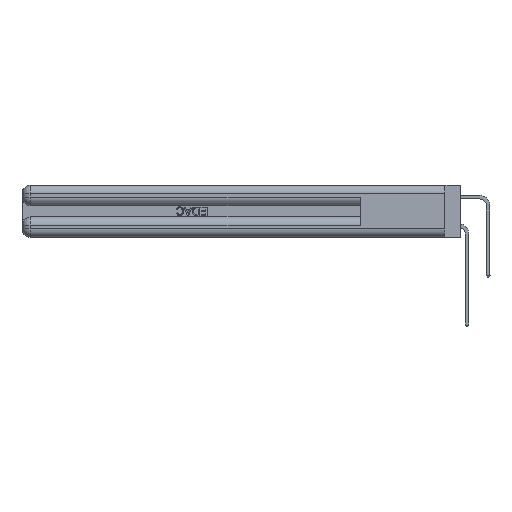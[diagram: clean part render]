
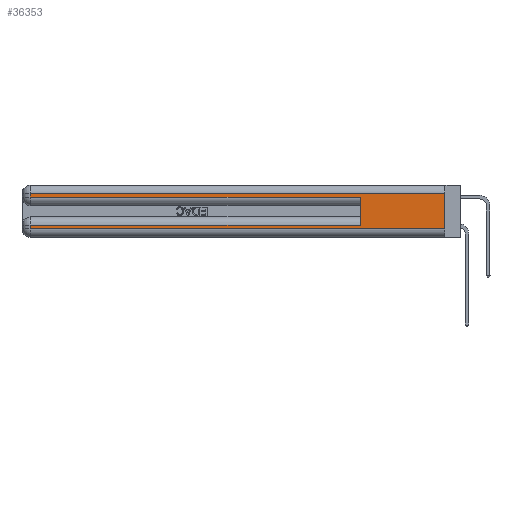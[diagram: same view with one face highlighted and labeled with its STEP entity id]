
A CAD part, left-side view. The second image highlights one B-rep face of the part: STEP entity #36353.
In plain terms, the highlighted planar face has unit normal (-1, 0, 0).
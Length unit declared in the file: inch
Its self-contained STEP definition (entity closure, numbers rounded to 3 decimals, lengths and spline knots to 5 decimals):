
#193 = CARTESIAN_POINT ( 'NONE',  ( 0., 0., 0.285 ) ) ;
#205 = EDGE_CURVE ( 'NONE', #13662, #18976, #2060, .T. ) ;
#457 = EDGE_CURVE ( 'NONE', #8145, #7969, #22100, .T. ) ;
#627 = DIRECTION ( 'NONE',  ( 0., 0., -1. ) ) ;
#692 = CARTESIAN_POINT ( 'NONE',  ( 0., 2.94, 0.37 ) ) ;
#2060 = LINE ( 'NONE', #39021, #38018 ) ;
#2291 = EDGE_CURVE ( 'NONE', #34204, #13143, #17756, .T. ) ;
#3431 = LINE ( 'NONE', #31493, #22983 ) ;
#3568 = LINE ( 'NONE', #34384, #14178 ) ;
#5233 = ORIENTED_EDGE ( 'NONE', *, *, #41923, .T. ) ;
#5401 = ORIENTED_EDGE ( 'NONE', *, *, #205, .T. ) ;
#5977 = DIRECTION ( 'NONE',  ( 0., 0., -1. ) ) ;
#6338 = ORIENTED_EDGE ( 'NONE', *, *, #2291, .F. ) ;
#6559 = EDGE_LOOP ( 'NONE', ( #21436, #18140, #39024, #5233, #6338, #36258, #5401, #8361 ) ) ;
#7005 = DIRECTION ( 'NONE',  ( 0., 1., 0. ) ) ;
#7896 = LINE ( 'NONE', #692, #8948 ) ;
#7969 = VERTEX_POINT ( 'NONE', #29337 ) ;
#8145 = VERTEX_POINT ( 'NONE', #39425 ) ;
#8361 = ORIENTED_EDGE ( 'NONE', *, *, #10549, .T. ) ;
#8948 = VECTOR ( 'NONE', #37995, 39.37008 ) ;
#9521 = CARTESIAN_POINT ( 'NONE',  ( 0., 0., 0.37 ) ) ;
#9901 = CARTESIAN_POINT ( 'NONE',  ( 0., 0.6, 0.145 ) ) ;
#10384 = FACE_OUTER_BOUND ( 'NONE', #6559, .T. ) ;
#10549 = EDGE_CURVE ( 'NONE', #18976, #26614, #3431, .T. ) ;
#13143 = VERTEX_POINT ( 'NONE', #22701 ) ;
#13662 = VERTEX_POINT ( 'NONE', #36046 ) ;
#14178 = VECTOR ( 'NONE', #7005, 39.37008 ) ;
#15717 = AXIS2_PLACEMENT_3D ( 'NONE', #9521, #23370, #5977 ) ;
#16528 = EDGE_CURVE ( 'NONE', #8145, #26614, #27671, .T. ) ;
#17756 = LINE ( 'NONE', #9901, #34706 ) ;
#18140 = ORIENTED_EDGE ( 'NONE', *, *, #457, .T. ) ;
#18976 = VERTEX_POINT ( 'NONE', #35636 ) ;
#19395 = EDGE_CURVE ( 'NONE', #7969, #34662, #7896, .T. ) ;
#19856 = EDGE_CURVE ( 'NONE', #34204, #13662, #3568, .T. ) ;
#21436 = ORIENTED_EDGE ( 'NONE', *, *, #16528, .F. ) ;
#21649 = CARTESIAN_POINT ( 'NONE',  ( 0., 0., 0.06 ) ) ;
#22033 = VECTOR ( 'NONE', #23367, 39.37008 ) ;
#22100 = LINE ( 'NONE', #36299, #41698 ) ;
#22149 = CARTESIAN_POINT ( 'NONE',  ( 0., 0., 0.37 ) ) ;
#22701 = CARTESIAN_POINT ( 'NONE',  ( 0., 0.6, 0.285 ) ) ;
#22983 = VECTOR ( 'NONE', #38126, 39.37008 ) ;
#23367 = DIRECTION ( 'NONE',  ( 0., -1., 0. ) ) ;
#23370 = DIRECTION ( 'NONE',  ( 1., 0., 0. ) ) ;
#26427 = DIRECTION ( 'NONE',  ( 0., 1., 0. ) ) ;
#26614 = VERTEX_POINT ( 'NONE', #21649 ) ;
#27671 = LINE ( 'NONE', #22149, #40911 ) ;
#28400 = LINE ( 'NONE', #193, #22033 ) ;
#29337 = CARTESIAN_POINT ( 'NONE',  ( 0., 2.94, 0.31 ) ) ;
#31493 = CARTESIAN_POINT ( 'NONE',  ( 0., 0., 0.06 ) ) ;
#31574 = CARTESIAN_POINT ( 'NONE',  ( 0., 0.6, 0.085 ) ) ;
#33456 = DIRECTION ( 'NONE',  ( 0., 0., 1. ) ) ;
#34204 = VERTEX_POINT ( 'NONE', #31574 ) ;
#34320 = CARTESIAN_POINT ( 'NONE',  ( 0., 2.94, 0.285 ) ) ;
#34384 = CARTESIAN_POINT ( 'NONE',  ( 0., 0., 0.085 ) ) ;
#34662 = VERTEX_POINT ( 'NONE', #34320 ) ;
#34706 = VECTOR ( 'NONE', #33456, 39.37008 ) ;
#35636 = CARTESIAN_POINT ( 'NONE',  ( 0., 2.94, 0.06 ) ) ;
#36046 = CARTESIAN_POINT ( 'NONE',  ( 0., 2.94, 0.085 ) ) ;
#36258 = ORIENTED_EDGE ( 'NONE', *, *, #19856, .T. ) ;
#36299 = CARTESIAN_POINT ( 'NONE',  ( 0., 0., 0.31 ) ) ;
#36353 = ADVANCED_FACE ( 'NONE', ( #10384 ), #36671, .F. ) ;
#36671 = PLANE ( 'NONE',  #15717 ) ;
#37995 = DIRECTION ( 'NONE',  ( 0., 0., -1. ) ) ;
#38018 = VECTOR ( 'NONE', #41235, 39.37008 ) ;
#38126 = DIRECTION ( 'NONE',  ( 0., -1., 0. ) ) ;
#39021 = CARTESIAN_POINT ( 'NONE',  ( 0., 2.94, 0.37 ) ) ;
#39024 = ORIENTED_EDGE ( 'NONE', *, *, #19395, .T. ) ;
#39425 = CARTESIAN_POINT ( 'NONE',  ( 0., 0., 0.31 ) ) ;
#40911 = VECTOR ( 'NONE', #627, 39.37008 ) ;
#41235 = DIRECTION ( 'NONE',  ( 0., 0., -1. ) ) ;
#41698 = VECTOR ( 'NONE', #26427, 39.37008 ) ;
#41923 = EDGE_CURVE ( 'NONE', #34662, #13143, #28400, .T. ) ;
